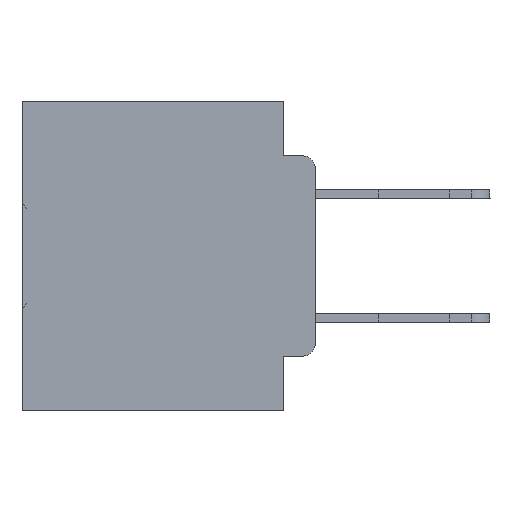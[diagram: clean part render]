
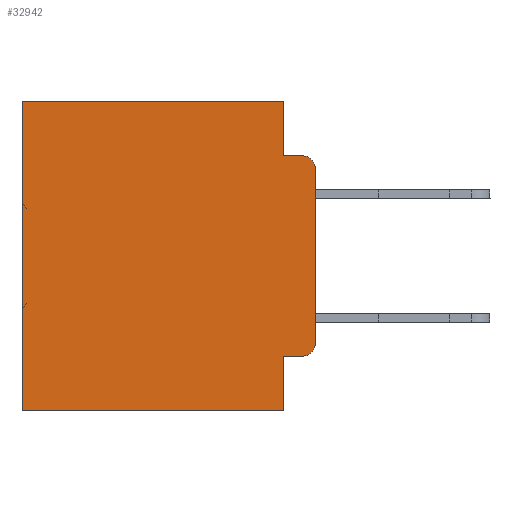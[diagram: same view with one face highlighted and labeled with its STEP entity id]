
A CAD part, left-side view. The second image highlights one B-rep face of the part: STEP entity #32942.
In plain terms, the highlighted planar face has unit normal (-1, 0, 0).
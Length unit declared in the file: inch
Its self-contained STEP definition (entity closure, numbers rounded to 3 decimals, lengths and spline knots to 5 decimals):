
#731 = CIRCLE ( 'NONE', #4372, 0.02 ) ;
#1355 = LINE ( 'NONE', #13034, #14957 ) ;
#1493 = VECTOR ( 'NONE', #15151, 39.37008 ) ;
#2223 = DIRECTION ( 'NONE',  ( 0., 0., -1. ) ) ;
#2470 = EDGE_CURVE ( 'NONE', #11007, #12761, #10730, .T. ) ;
#2841 = CARTESIAN_POINT ( 'NONE',  ( 0.298, 0.473, -0.5 ) ) ;
#2908 = EDGE_CURVE ( 'NONE', #12761, #21565, #19214, .T. ) ;
#3282 = EDGE_CURVE ( 'NONE', #19229, #11365, #36247, .T. ) ;
#3462 = CARTESIAN_POINT ( 'NONE',  ( 0.298, 0., 0. ) ) ;
#3473 = CARTESIAN_POINT ( 'NONE',  ( 0.298, 0., -0.5 ) ) ;
#3542 = DIRECTION ( 'NONE',  ( 0., -1., 0. ) ) ;
#4372 = AXIS2_PLACEMENT_3D ( 'NONE', #32878, #23514, #32318 ) ;
#4513 = ORIENTED_EDGE ( 'NONE', *, *, #24484, .F. ) ;
#4756 = VERTEX_POINT ( 'NONE', #23616 ) ;
#4975 = CARTESIAN_POINT ( 'NONE',  ( 0.298, 0.473, 0. ) ) ;
#4977 = VECTOR ( 'NONE', #36060, 39.37008 ) ;
#5091 = CARTESIAN_POINT ( 'NONE',  ( 0.298, 0.02, -0.3915 ) ) ;
#6758 = CARTESIAN_POINT ( 'NONE',  ( 0.298, 0.02, -0.0885 ) ) ;
#6923 = ORIENTED_EDGE ( 'NONE', *, *, #27527, .F. ) ;
#7233 = EDGE_CURVE ( 'NONE', #4756, #10665, #25605, .T. ) ;
#9170 = AXIS2_PLACEMENT_3D ( 'NONE', #28492, #25812, #28308 ) ;
#9483 = VERTEX_POINT ( 'NONE', #13403 ) ;
#9578 = LINE ( 'NONE', #3462, #25647 ) ;
#9701 = VECTOR ( 'NONE', #33701, 39.37008 ) ;
#10419 = LINE ( 'NONE', #24577, #36148 ) ;
#10665 = VERTEX_POINT ( 'NONE', #6758 ) ;
#10730 = LINE ( 'NONE', #34081, #9701 ) ;
#11007 = VERTEX_POINT ( 'NONE', #37749 ) ;
#11365 = VERTEX_POINT ( 'NONE', #4975 ) ;
#11515 = DIRECTION ( 'NONE',  ( 0., 0., -1. ) ) ;
#12664 = CARTESIAN_POINT ( 'NONE',  ( 0.298, 0.051, -0.5 ) ) ;
#12717 = VERTEX_POINT ( 'NONE', #12664 ) ;
#12761 = VERTEX_POINT ( 'NONE', #20892 ) ;
#12998 = EDGE_CURVE ( 'NONE', #11007, #12717, #1355, .T. ) ;
#13034 = CARTESIAN_POINT ( 'NONE',  ( 0.298, 0.051, 0. ) ) ;
#13403 = CARTESIAN_POINT ( 'NONE',  ( 0.298, 0., -0.1085 ) ) ;
#14957 = VECTOR ( 'NONE', #24692, 39.37008 ) ;
#15151 = DIRECTION ( 'NONE',  ( 0., 1., 0. ) ) ;
#16204 = ORIENTED_EDGE ( 'NONE', *, *, #34641, .T. ) ;
#16465 = FACE_OUTER_BOUND ( 'NONE', #17828, .T. ) ;
#16746 = DIRECTION ( 'NONE',  ( 0., 0., -1. ) ) ;
#17084 = LINE ( 'NONE', #26042, #32353 ) ;
#17118 = ORIENTED_EDGE ( 'NONE', *, *, #17534, .F. ) ;
#17347 = DIRECTION ( 'NONE',  ( -1., 0., 0. ) ) ;
#17534 = EDGE_CURVE ( 'NONE', #12717, #22145, #32366, .T. ) ;
#17739 = VECTOR ( 'NONE', #3542, 39.37008 ) ;
#17828 = EDGE_LOOP ( 'NONE', ( #4513, #16204, #21660, #6923, #21015, #17906, #17118, #22975, #24950, #32979 ) ) ;
#17906 = ORIENTED_EDGE ( 'NONE', *, *, #32487, .T. ) ;
#18090 = CARTESIAN_POINT ( 'NONE',  ( 0.298, 0.051, -0.0885 ) ) ;
#18383 = DIRECTION ( 'NONE',  ( 0., 0., -1. ) ) ;
#18606 = AXIS2_PLACEMENT_3D ( 'NONE', #5091, #17347, #2223 ) ;
#18786 = CARTESIAN_POINT ( 'NONE',  ( 0.298, 0., -0.3915 ) ) ;
#19214 = CIRCLE ( 'NONE', #18606, 0.02 ) ;
#19229 = VERTEX_POINT ( 'NONE', #26765 ) ;
#20892 = CARTESIAN_POINT ( 'NONE',  ( 0.298, 0.02, -0.4115 ) ) ;
#21015 = ORIENTED_EDGE ( 'NONE', *, *, #3282, .T. ) ;
#21565 = VERTEX_POINT ( 'NONE', #18786 ) ;
#21660 = ORIENTED_EDGE ( 'NONE', *, *, #7233, .F. ) ;
#22145 = VERTEX_POINT ( 'NONE', #2841 ) ;
#22975 = ORIENTED_EDGE ( 'NONE', *, *, #12998, .F. ) ;
#23514 = DIRECTION ( 'NONE',  ( -1., 0., 0. ) ) ;
#23616 = CARTESIAN_POINT ( 'NONE',  ( 0.298, 0.051, -0.0885 ) ) ;
#24484 = EDGE_CURVE ( 'NONE', #9483, #21565, #9578, .T. ) ;
#24577 = CARTESIAN_POINT ( 'NONE',  ( 0.298, 0.051, 0. ) ) ;
#24692 = DIRECTION ( 'NONE',  ( 0., 0., -1. ) ) ;
#24950 = ORIENTED_EDGE ( 'NONE', *, *, #2470, .T. ) ;
#25605 = LINE ( 'NONE', #18090, #17739 ) ;
#25647 = VECTOR ( 'NONE', #18383, 39.37008 ) ;
#25812 = DIRECTION ( 'NONE',  ( 1., 0., 0. ) ) ;
#26042 = CARTESIAN_POINT ( 'NONE',  ( 0.298, 0.473, 0. ) ) ;
#26765 = CARTESIAN_POINT ( 'NONE',  ( 0.298, 0.051, 0. ) ) ;
#27527 = EDGE_CURVE ( 'NONE', #19229, #4756, #10419, .T. ) ;
#28120 = PLANE ( 'NONE',  #9170 ) ;
#28308 = DIRECTION ( 'NONE',  ( 0., 0., -1. ) ) ;
#28492 = CARTESIAN_POINT ( 'NONE',  ( 0.298, 0., 0. ) ) ;
#32318 = DIRECTION ( 'NONE',  ( 0., 0., -1. ) ) ;
#32353 = VECTOR ( 'NONE', #11515, 39.37008 ) ;
#32366 = LINE ( 'NONE', #3473, #1493 ) ;
#32487 = EDGE_CURVE ( 'NONE', #11365, #22145, #17084, .T. ) ;
#32878 = CARTESIAN_POINT ( 'NONE',  ( 0.298, 0.02, -0.1085 ) ) ;
#32942 = ADVANCED_FACE ( 'NONE', ( #16465 ), #28120, .F. ) ;
#32979 = ORIENTED_EDGE ( 'NONE', *, *, #2908, .T. ) ;
#33701 = DIRECTION ( 'NONE',  ( 0., -1., 0. ) ) ;
#34081 = CARTESIAN_POINT ( 'NONE',  ( 0.298, 0.051, -0.4115 ) ) ;
#34641 = EDGE_CURVE ( 'NONE', #9483, #10665, #731, .T. ) ;
#36060 = DIRECTION ( 'NONE',  ( 0., 1., 0. ) ) ;
#36148 = VECTOR ( 'NONE', #16746, 39.37008 ) ;
#36247 = LINE ( 'NONE', #36623, #4977 ) ;
#36623 = CARTESIAN_POINT ( 'NONE',  ( 0.298, 0., 0. ) ) ;
#37749 = CARTESIAN_POINT ( 'NONE',  ( 0.298, 0.051, -0.4115 ) ) ;
